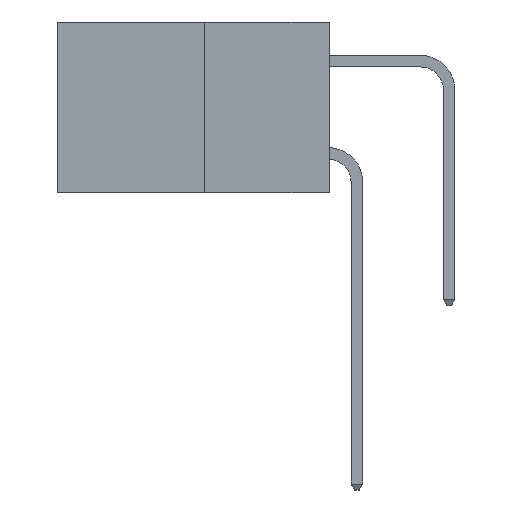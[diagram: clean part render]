
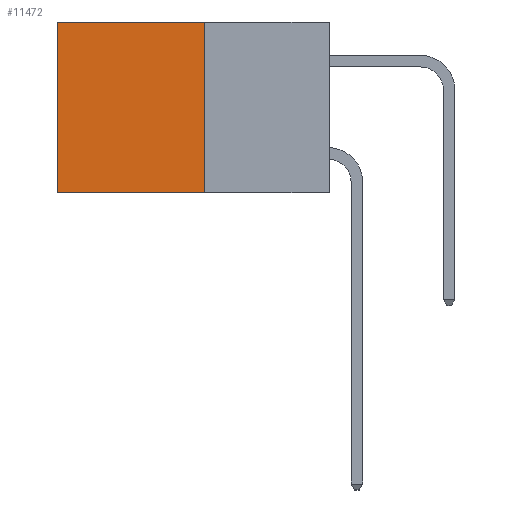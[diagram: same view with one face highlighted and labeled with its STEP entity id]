
A CAD part, left-side view. The second image highlights one B-rep face of the part: STEP entity #11472.
In plain terms, the highlighted planar face has unit normal (-1, 0, 0).
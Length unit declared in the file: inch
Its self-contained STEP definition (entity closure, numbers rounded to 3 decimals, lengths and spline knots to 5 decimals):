
#6 = DIRECTION ( 'NONE',  ( 1., 0., 0. ) ) ;
#209 = CARTESIAN_POINT ( 'NONE',  ( 0.277, 0.27, -0.37 ) ) ;
#646 = LINE ( 'NONE', #10167, #10899 ) ;
#1226 = LINE ( 'NONE', #11971, #3518 ) ;
#1305 = FACE_OUTER_BOUND ( 'NONE', #12003, .T. ) ;
#2587 = VECTOR ( 'NONE', #11790, 39.37008 ) ;
#3463 = ORIENTED_EDGE ( 'NONE', *, *, #8278, .T. ) ;
#3518 = VECTOR ( 'NONE', #4361, 39.37008 ) ;
#3943 = VECTOR ( 'NONE', #10080, 39.37008 ) ;
#4361 = DIRECTION ( 'NONE',  ( 0., 1., 0. ) ) ;
#4418 = DIRECTION ( 'NONE',  ( 0., 0., -1. ) ) ;
#5620 = VERTEX_POINT ( 'NONE', #209 ) ;
#5667 = VERTEX_POINT ( 'NONE', #9018 ) ;
#5681 = EDGE_CURVE ( 'NONE', #6336, #5620, #12166, .T. ) ;
#5839 = EDGE_CURVE ( 'NONE', #8556, #5667, #646, .T. ) ;
#6336 = VERTEX_POINT ( 'NONE', #9004 ) ;
#6765 = PLANE ( 'NONE',  #9934 ) ;
#6844 = DIRECTION ( 'NONE',  ( 0., 0., -1. ) ) ;
#7813 = ORIENTED_EDGE ( 'NONE', *, *, #5839, .T. ) ;
#8278 = EDGE_CURVE ( 'NONE', #6336, #8556, #9681, .T. ) ;
#8340 = ORIENTED_EDGE ( 'NONE', *, *, #9007, .F. ) ;
#8556 = VERTEX_POINT ( 'NONE', #9537 ) ;
#9004 = CARTESIAN_POINT ( 'NONE',  ( 0.277, 0.27, 0. ) ) ;
#9007 = EDGE_CURVE ( 'NONE', #5620, #5667, #1226, .T. ) ;
#9018 = CARTESIAN_POINT ( 'NONE',  ( 0.277, 0.59, -0.37 ) ) ;
#9217 = CARTESIAN_POINT ( 'NONE',  ( 0.277, 0.27, 0. ) ) ;
#9537 = CARTESIAN_POINT ( 'NONE',  ( 0.277, 0.59, 0. ) ) ;
#9635 = ORIENTED_EDGE ( 'NONE', *, *, #5681, .F. ) ;
#9681 = LINE ( 'NONE', #9217, #3943 ) ;
#9934 = AXIS2_PLACEMENT_3D ( 'NONE', #11530, #6, #6844 ) ;
#10080 = DIRECTION ( 'NONE',  ( 0., 1., 0. ) ) ;
#10167 = CARTESIAN_POINT ( 'NONE',  ( 0.277, 0.59, -0.37 ) ) ;
#10869 = CARTESIAN_POINT ( 'NONE',  ( 0.277, 0.27, -0.37 ) ) ;
#10899 = VECTOR ( 'NONE', #4418, 39.37008 ) ;
#11472 = ADVANCED_FACE ( 'NONE', ( #1305 ), #6765, .F. ) ;
#11530 = CARTESIAN_POINT ( 'NONE',  ( 0.277, 0.27, -0.37 ) ) ;
#11790 = DIRECTION ( 'NONE',  ( 0., 0., -1. ) ) ;
#11971 = CARTESIAN_POINT ( 'NONE',  ( 0.277, 0.27, -0.37 ) ) ;
#12003 = EDGE_LOOP ( 'NONE', ( #7813, #8340, #9635, #3463 ) ) ;
#12166 = LINE ( 'NONE', #10869, #2587 ) ;
